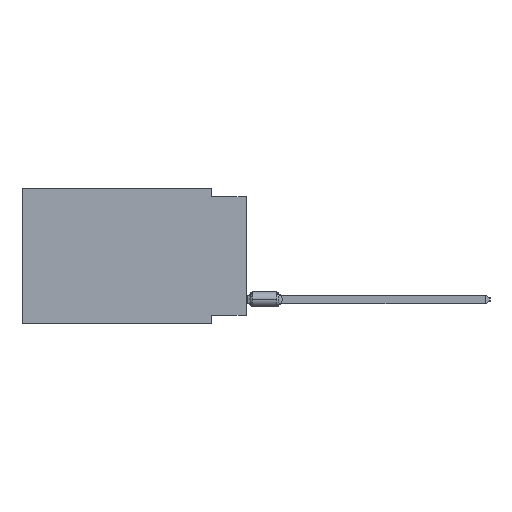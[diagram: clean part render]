
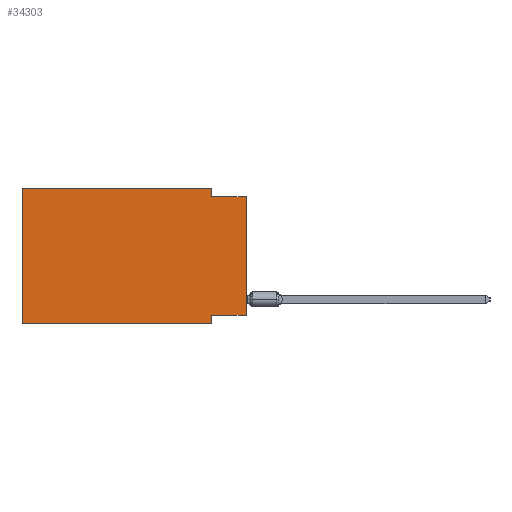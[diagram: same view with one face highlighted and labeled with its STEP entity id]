
A CAD part, left-side view. The second image highlights one B-rep face of the part: STEP entity #34303.
In plain terms, the highlighted planar face has unit normal (-1, 0, 0).
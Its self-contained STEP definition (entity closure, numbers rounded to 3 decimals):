
#55 = DIRECTION ( 'NONE',  ( 0., 1., 0. ) ) ;
#1503 = VERTEX_POINT ( 'NONE', #8014 ) ;
#2741 = VERTEX_POINT ( 'NONE', #13649 ) ;
#3794 = EDGE_CURVE ( 'NONE', #32915, #47426, #47769, .T. ) ;
#3829 = DIRECTION ( 'NONE',  ( 0., -1., 0. ) ) ;
#4109 = EDGE_CURVE ( 'NONE', #21044, #23647, #57325, .T. ) ;
#4355 = DIRECTION ( 'NONE',  ( 0., -1., 0. ) ) ;
#4488 = VECTOR ( 'NONE', #55, 1000. ) ;
#4559 = CARTESIAN_POINT ( 'NONE',  ( 0., 16.383, 0. ) ) ;
#7923 = AXIS2_PLACEMENT_3D ( 'NONE', #14432, #58018, #8912 ) ;
#8014 = CARTESIAN_POINT ( 'NONE',  ( 0., 16.383, -9.906 ) ) ;
#8723 = LINE ( 'NONE', #36410, #32831 ) ;
#8912 = DIRECTION ( 'NONE',  ( 0., 0., -1. ) ) ;
#9090 = ORIENTED_EDGE ( 'NONE', *, *, #33268, .F. ) ;
#9216 = DIRECTION ( 'NONE',  ( 0., 0., -1. ) ) ;
#11011 = VERTEX_POINT ( 'NONE', #40541 ) ;
#12263 = VECTOR ( 'NONE', #40342, 1000. ) ;
#13061 = ORIENTED_EDGE ( 'NONE', *, *, #4109, .T. ) ;
#13399 = CARTESIAN_POINT ( 'NONE',  ( 0., 2.54, -9.271 ) ) ;
#13649 = CARTESIAN_POINT ( 'NONE',  ( 0., 2.54, -9.906 ) ) ;
#13688 = ORIENTED_EDGE ( 'NONE', *, *, #24347, .F. ) ;
#13721 = LINE ( 'NONE', #26613, #20600 ) ;
#14240 = DIRECTION ( 'NONE',  ( 0., -1., 0. ) ) ;
#14432 = CARTESIAN_POINT ( 'NONE',  ( 0., 16.383, 0. ) ) ;
#15411 = LINE ( 'NONE', #32396, #30267 ) ;
#18294 = EDGE_CURVE ( 'NONE', #1503, #32915, #39469, .T. ) ;
#18670 = CARTESIAN_POINT ( 'NONE',  ( 0., 0., -0.635 ) ) ;
#18698 = CARTESIAN_POINT ( 'NONE',  ( 0., 0., -9.271 ) ) ;
#18869 = FACE_OUTER_BOUND ( 'NONE', #20553, .T. ) ;
#20200 = EDGE_CURVE ( 'NONE', #47426, #11011, #13721, .T. ) ;
#20553 = EDGE_LOOP ( 'NONE', ( #13061, #58463, #61745, #58123, #52975, #38424, #9090, #13688 ) ) ;
#20600 = VECTOR ( 'NONE', #70221, 1000. ) ;
#21044 = VERTEX_POINT ( 'NONE', #18698 ) ;
#23647 = VERTEX_POINT ( 'NONE', #18670 ) ;
#23873 = VECTOR ( 'NONE', #46084, 1000. ) ;
#24347 = EDGE_CURVE ( 'NONE', #21044, #63945, #67300, .T. ) ;
#26613 = CARTESIAN_POINT ( 'NONE',  ( 0., 2.54, 0. ) ) ;
#30267 = VECTOR ( 'NONE', #4355, 1000. ) ;
#32396 = CARTESIAN_POINT ( 'NONE',  ( 0., 0., -0.635 ) ) ;
#32831 = VECTOR ( 'NONE', #14240, 1000. ) ;
#32915 = VERTEX_POINT ( 'NONE', #4559 ) ;
#33268 = EDGE_CURVE ( 'NONE', #63945, #2741, #64975, .T. ) ;
#34066 = CARTESIAN_POINT ( 'NONE',  ( 0., 0., 0. ) ) ;
#34303 = ADVANCED_FACE ( 'NONE', ( #18869 ), #63934, .F. ) ;
#36410 = CARTESIAN_POINT ( 'NONE',  ( 0., 16.383, -9.906 ) ) ;
#38182 = VECTOR ( 'NONE', #3829, 1000. ) ;
#38424 = ORIENTED_EDGE ( 'NONE', *, *, #44550, .T. ) ;
#39469 = LINE ( 'NONE', #46441, #23873 ) ;
#40342 = DIRECTION ( 'NONE',  ( 0., 0., 1. ) ) ;
#40347 = CARTESIAN_POINT ( 'NONE',  ( 0., 2.54, -9.906 ) ) ;
#40541 = CARTESIAN_POINT ( 'NONE',  ( 0., 2.54, -0.635 ) ) ;
#44550 = EDGE_CURVE ( 'NONE', #1503, #2741, #8723, .T. ) ;
#46084 = DIRECTION ( 'NONE',  ( 0., 0., 1. ) ) ;
#46441 = CARTESIAN_POINT ( 'NONE',  ( 0., 16.383, 0. ) ) ;
#47426 = VERTEX_POINT ( 'NONE', #53718 ) ;
#47769 = LINE ( 'NONE', #53686, #38182 ) ;
#52975 = ORIENTED_EDGE ( 'NONE', *, *, #18294, .F. ) ;
#53686 = CARTESIAN_POINT ( 'NONE',  ( 0., 16.383, 0. ) ) ;
#53718 = CARTESIAN_POINT ( 'NONE',  ( 0., 2.54, 0. ) ) ;
#56146 = VECTOR ( 'NONE', #9216, 1000. ) ;
#57325 = LINE ( 'NONE', #34066, #12263 ) ;
#58018 = DIRECTION ( 'NONE',  ( 1., 0., 0. ) ) ;
#58123 = ORIENTED_EDGE ( 'NONE', *, *, #3794, .F. ) ;
#58463 = ORIENTED_EDGE ( 'NONE', *, *, #71731, .F. ) ;
#61745 = ORIENTED_EDGE ( 'NONE', *, *, #20200, .F. ) ;
#61757 = CARTESIAN_POINT ( 'NONE',  ( 0., 0., -9.271 ) ) ;
#63934 = PLANE ( 'NONE',  #7923 ) ;
#63945 = VERTEX_POINT ( 'NONE', #13399 ) ;
#64975 = LINE ( 'NONE', #40347, #56146 ) ;
#67300 = LINE ( 'NONE', #61757, #4488 ) ;
#70221 = DIRECTION ( 'NONE',  ( 0., 0., -1. ) ) ;
#71731 = EDGE_CURVE ( 'NONE', #11011, #23647, #15411, .T. ) ;
